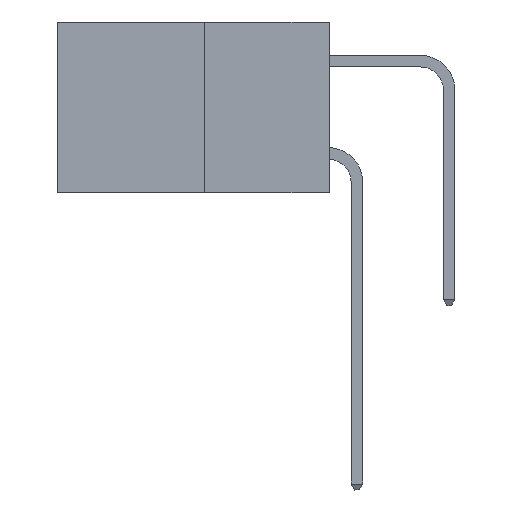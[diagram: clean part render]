
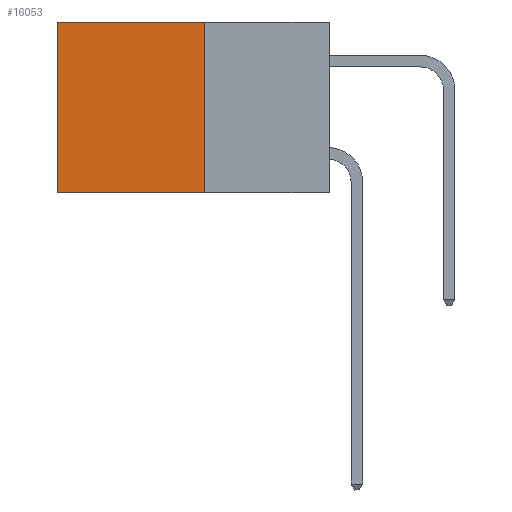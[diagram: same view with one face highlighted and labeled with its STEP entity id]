
A CAD part, left-side view. The second image highlights one B-rep face of the part: STEP entity #16053.
In plain terms, the highlighted planar face has unit normal (-1, 0, 0).
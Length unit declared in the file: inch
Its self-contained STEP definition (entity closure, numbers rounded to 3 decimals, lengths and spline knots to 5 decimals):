
#436 = VERTEX_POINT ( 'NONE', #25589 ) ;
#2101 = ORIENTED_EDGE ( 'NONE', *, *, #15037, .T. ) ;
#3314 = CARTESIAN_POINT ( 'NONE',  ( 0.277, 0.27, 0. ) ) ;
#3561 = VECTOR ( 'NONE', #22537, 39.37008 ) ;
#4139 = LINE ( 'NONE', #15120, #19492 ) ;
#4318 = DIRECTION ( 'NONE',  ( 0., 0., -1. ) ) ;
#6448 = CARTESIAN_POINT ( 'NONE',  ( 0.277, 0.27, -0.37 ) ) ;
#7435 = CARTESIAN_POINT ( 'NONE',  ( 0.277, 0.27, 0. ) ) ;
#8122 = LINE ( 'NONE', #7435, #3561 ) ;
#8752 = FACE_OUTER_BOUND ( 'NONE', #16367, .T. ) ;
#9039 = CARTESIAN_POINT ( 'NONE',  ( 0.277, 0.27, -0.37 ) ) ;
#9156 = CARTESIAN_POINT ( 'NONE',  ( 0.277, 0.59, 0. ) ) ;
#9720 = CARTESIAN_POINT ( 'NONE',  ( 0.277, 0.59, -0.37 ) ) ;
#9745 = EDGE_CURVE ( 'NONE', #436, #26852, #4139, .T. ) ;
#11241 = PLANE ( 'NONE',  #13960 ) ;
#11993 = DIRECTION ( 'NONE',  ( 0., 0., -1. ) ) ;
#12705 = EDGE_CURVE ( 'NONE', #15179, #436, #26005, .T. ) ;
#13371 = DIRECTION ( 'NONE',  ( 0., 0., -1. ) ) ;
#13960 = AXIS2_PLACEMENT_3D ( 'NONE', #9039, #26168, #13371 ) ;
#14449 = CARTESIAN_POINT ( 'NONE',  ( 0.277, 0.59, -0.37 ) ) ;
#15009 = ORIENTED_EDGE ( 'NONE', *, *, #17606, .T. ) ;
#15037 = EDGE_CURVE ( 'NONE', #15179, #23446, #8122, .T. ) ;
#15120 = CARTESIAN_POINT ( 'NONE',  ( 0.277, 0.27, -0.37 ) ) ;
#15179 = VERTEX_POINT ( 'NONE', #3314 ) ;
#15189 = ORIENTED_EDGE ( 'NONE', *, *, #9745, .F. ) ;
#16053 = ADVANCED_FACE ( 'NONE', ( #8752 ), #11241, .F. ) ;
#16367 = EDGE_LOOP ( 'NONE', ( #15009, #15189, #22283, #2101 ) ) ;
#17606 = EDGE_CURVE ( 'NONE', #23446, #26852, #24770, .T. ) ;
#19141 = VECTOR ( 'NONE', #11993, 39.37008 ) ;
#19492 = VECTOR ( 'NONE', #25695, 39.37008 ) ;
#19721 = VECTOR ( 'NONE', #4318, 39.37008 ) ;
#22283 = ORIENTED_EDGE ( 'NONE', *, *, #12705, .F. ) ;
#22537 = DIRECTION ( 'NONE',  ( 0., 1., 0. ) ) ;
#23446 = VERTEX_POINT ( 'NONE', #9156 ) ;
#24770 = LINE ( 'NONE', #9720, #19141 ) ;
#25589 = CARTESIAN_POINT ( 'NONE',  ( 0.277, 0.27, -0.37 ) ) ;
#25695 = DIRECTION ( 'NONE',  ( 0., 1., 0. ) ) ;
#26005 = LINE ( 'NONE', #6448, #19721 ) ;
#26168 = DIRECTION ( 'NONE',  ( 1., 0., 0. ) ) ;
#26852 = VERTEX_POINT ( 'NONE', #14449 ) ;
